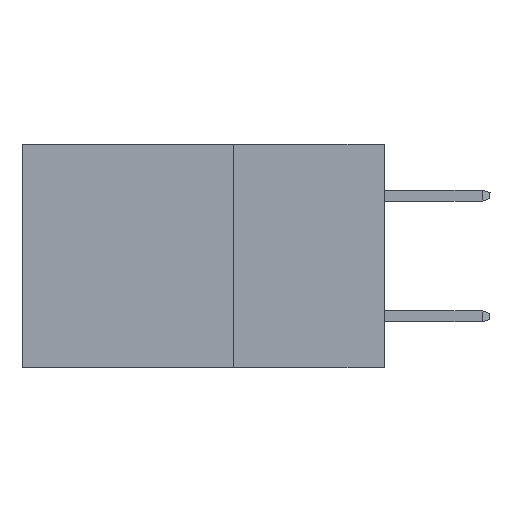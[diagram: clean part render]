
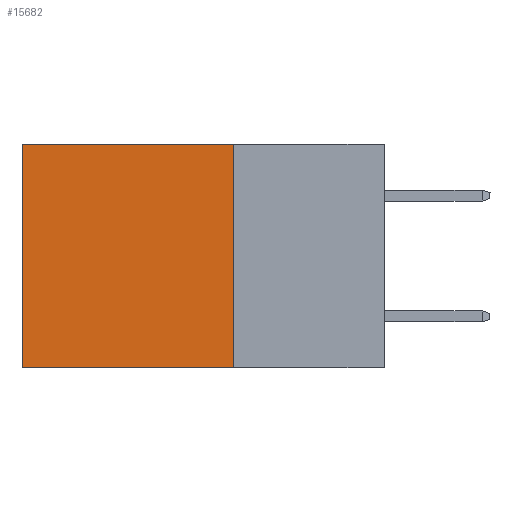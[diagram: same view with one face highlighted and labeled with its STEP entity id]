
A CAD part, left-side view. The second image highlights one B-rep face of the part: STEP entity #15682.
In plain terms, the highlighted planar face has unit normal (-1, 0, 0).
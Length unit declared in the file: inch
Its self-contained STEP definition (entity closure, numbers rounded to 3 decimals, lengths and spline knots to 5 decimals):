
#32 = ORIENTED_EDGE ( 'NONE', *, *, #2495, .T. ) ;
#572 = CARTESIAN_POINT ( 'NONE',  ( 0.298, 0.6, -0.37 ) ) ;
#644 = VERTEX_POINT ( 'NONE', #15123 ) ;
#700 = CARTESIAN_POINT ( 'NONE',  ( 0.298, 0.25, 0. ) ) ;
#1364 = LINE ( 'NONE', #1945, #9138 ) ;
#1498 = VERTEX_POINT ( 'NONE', #572 ) ;
#1945 = CARTESIAN_POINT ( 'NONE',  ( 0.298, 0.25, 0. ) ) ;
#2126 = CARTESIAN_POINT ( 'NONE',  ( 0.298, 0.25, 0. ) ) ;
#2267 = EDGE_CURVE ( 'NONE', #644, #1498, #7094, .T. ) ;
#2495 = EDGE_CURVE ( 'NONE', #9385, #1498, #6151, .T. ) ;
#2811 = DIRECTION ( 'NONE',  ( 0., 1., 0. ) ) ;
#3067 = DIRECTION ( 'NONE',  ( 0., 0., -1. ) ) ;
#3088 = DIRECTION ( 'NONE',  ( 0., 0., -1. ) ) ;
#3690 = ORIENTED_EDGE ( 'NONE', *, *, #12589, .T. ) ;
#3919 = CARTESIAN_POINT ( 'NONE',  ( 0.298, 0.6, 0. ) ) ;
#4210 = AXIS2_PLACEMENT_3D ( 'NONE', #2126, #15474, #8246 ) ;
#4295 = DIRECTION ( 'NONE',  ( 0., 1., 0. ) ) ;
#5011 = CARTESIAN_POINT ( 'NONE',  ( 0.298, 0.25, -0.37 ) ) ;
#5484 = PLANE ( 'NONE',  #4210 ) ;
#5501 = FACE_OUTER_BOUND ( 'NONE', #9038, .T. ) ;
#6151 = LINE ( 'NONE', #10203, #12279 ) ;
#6929 = VECTOR ( 'NONE', #2811, 39.37008 ) ;
#7094 = LINE ( 'NONE', #5011, #7681 ) ;
#7323 = LINE ( 'NONE', #11506, #6929 ) ;
#7681 = VECTOR ( 'NONE', #4295, 39.37008 ) ;
#8246 = DIRECTION ( 'NONE',  ( 0., 0., -1. ) ) ;
#9038 = EDGE_LOOP ( 'NONE', ( #32, #10170, #15378, #3690 ) ) ;
#9138 = VECTOR ( 'NONE', #3067, 39.37008 ) ;
#9385 = VERTEX_POINT ( 'NONE', #3919 ) ;
#9540 = EDGE_CURVE ( 'NONE', #11333, #644, #1364, .T. ) ;
#10170 = ORIENTED_EDGE ( 'NONE', *, *, #2267, .F. ) ;
#10203 = CARTESIAN_POINT ( 'NONE',  ( 0.298, 0.6, 0. ) ) ;
#11333 = VERTEX_POINT ( 'NONE', #700 ) ;
#11506 = CARTESIAN_POINT ( 'NONE',  ( 0.298, 0.25, 0. ) ) ;
#12279 = VECTOR ( 'NONE', #3088, 39.37008 ) ;
#12589 = EDGE_CURVE ( 'NONE', #11333, #9385, #7323, .T. ) ;
#15123 = CARTESIAN_POINT ( 'NONE',  ( 0.298, 0.25, -0.37 ) ) ;
#15378 = ORIENTED_EDGE ( 'NONE', *, *, #9540, .F. ) ;
#15474 = DIRECTION ( 'NONE',  ( 1., 0., 0. ) ) ;
#15682 = ADVANCED_FACE ( 'NONE', ( #5501 ), #5484, .F. ) ;
